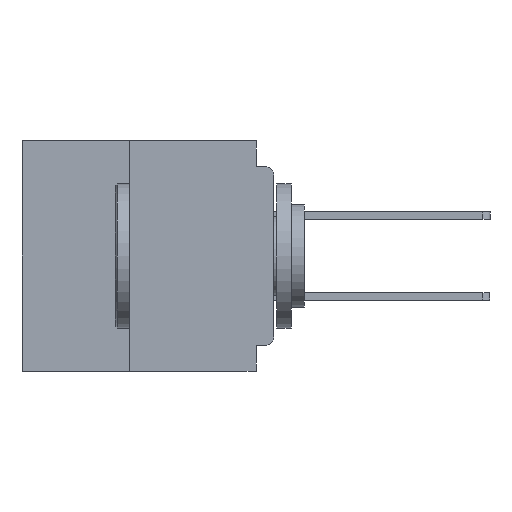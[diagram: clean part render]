
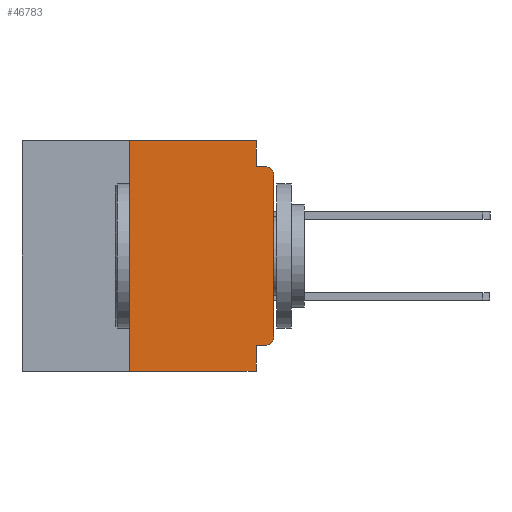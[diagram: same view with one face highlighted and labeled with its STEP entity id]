
A CAD part, left-side view. The second image highlights one B-rep face of the part: STEP entity #46783.
In plain terms, the highlighted planar face has unit normal (-1, 0, 0).
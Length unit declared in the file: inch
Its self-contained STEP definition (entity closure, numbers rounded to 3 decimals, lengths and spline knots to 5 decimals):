
#150 = VERTEX_POINT ( 'NONE', #36035 ) ;
#261 = ORIENTED_EDGE ( 'NONE', *, *, #5067, .T. ) ;
#636 = LINE ( 'NONE', #28807, #11610 ) ;
#663 = CARTESIAN_POINT ( 'NONE',  ( 0., 0.015, -0.355 ) ) ;
#1056 = CIRCLE ( 'NONE', #18691, 0.015 ) ;
#1163 = CIRCLE ( 'NONE', #52156, 0.015 ) ;
#1721 = ORIENTED_EDGE ( 'NONE', *, *, #18820, .F. ) ;
#1840 = LINE ( 'NONE', #54053, #12807 ) ;
#2618 = DIRECTION ( 'NONE',  ( 0., -1., 0. ) ) ;
#2851 = VERTEX_POINT ( 'NONE', #39978 ) ;
#3169 = DIRECTION ( 'NONE',  ( 0., 0., -1. ) ) ;
#3221 = VERTEX_POINT ( 'NONE', #18459 ) ;
#5067 = EDGE_CURVE ( 'NONE', #38964, #11904, #1056, .T. ) ;
#7493 = VECTOR ( 'NONE', #14672, 39.37008 ) ;
#8083 = LINE ( 'NONE', #48654, #31154 ) ;
#8415 = DIRECTION ( 'NONE',  ( 0., 0., -1. ) ) ;
#9556 = VERTEX_POINT ( 'NONE', #18477 ) ;
#10349 = EDGE_LOOP ( 'NONE', ( #28028, #261, #1721, #19710, #19076, #18080, #38736, #49837, #51034, #35666 ) ) ;
#10850 = EDGE_CURVE ( 'NONE', #9556, #2851, #44043, .T. ) ;
#11000 = VECTOR ( 'NONE', #44544, 39.37008 ) ;
#11610 = VECTOR ( 'NONE', #37905, 39.37008 ) ;
#11904 = VERTEX_POINT ( 'NONE', #25648 ) ;
#11950 = EDGE_CURVE ( 'NONE', #24018, #38964, #8083, .T. ) ;
#12476 = LINE ( 'NONE', #21723, #11000 ) ;
#12807 = VECTOR ( 'NONE', #8415, 39.37008 ) ;
#13900 = CARTESIAN_POINT ( 'NONE',  ( 0., 0.437, 0. ) ) ;
#14672 = DIRECTION ( 'NONE',  ( 0., 0., -1. ) ) ;
#15070 = VECTOR ( 'NONE', #2618, 39.37008 ) ;
#16464 = PLANE ( 'NONE',  #28823 ) ;
#16754 = VECTOR ( 'NONE', #18567, 39.37008 ) ;
#16931 = VERTEX_POINT ( 'NONE', #33832 ) ;
#18080 = ORIENTED_EDGE ( 'NONE', *, *, #25712, .F. ) ;
#18108 = DIRECTION ( 'NONE',  ( 0., 0., -1. ) ) ;
#18177 = DIRECTION ( 'NONE',  ( -1., 0., 0. ) ) ;
#18235 = CARTESIAN_POINT ( 'NONE',  ( 0., 0.015, -0.06 ) ) ;
#18459 = CARTESIAN_POINT ( 'NONE',  ( 0., 0.25, 0. ) ) ;
#18477 = CARTESIAN_POINT ( 'NONE',  ( 0., 0.031, 0. ) ) ;
#18567 = DIRECTION ( 'NONE',  ( 0., -1., 0. ) ) ;
#18691 = AXIS2_PLACEMENT_3D ( 'NONE', #18235, #18177, #18108 ) ;
#18820 = EDGE_CURVE ( 'NONE', #2851, #11904, #12476, .T. ) ;
#19076 = ORIENTED_EDGE ( 'NONE', *, *, #43792, .F. ) ;
#19710 = ORIENTED_EDGE ( 'NONE', *, *, #10850, .F. ) ;
#21723 = CARTESIAN_POINT ( 'NONE',  ( 0., 0., -0.045 ) ) ;
#21734 = CARTESIAN_POINT ( 'NONE',  ( 0., 0.031, -0.355 ) ) ;
#22183 = CARTESIAN_POINT ( 'NONE',  ( 0., 0., -0.06 ) ) ;
#24018 = VERTEX_POINT ( 'NONE', #51856 ) ;
#24829 = VERTEX_POINT ( 'NONE', #21734 ) ;
#25648 = CARTESIAN_POINT ( 'NONE',  ( 0., 0.015, -0.045 ) ) ;
#25712 = EDGE_CURVE ( 'NONE', #16931, #3221, #636, .T. ) ;
#26240 = DIRECTION ( 'NONE',  ( 0., 0., 1. ) ) ;
#26514 = DIRECTION ( 'NONE',  ( 0., 0., -1. ) ) ;
#27223 = EDGE_CURVE ( 'NONE', #24829, #150, #1840, .T. ) ;
#28028 = ORIENTED_EDGE ( 'NONE', *, *, #11950, .T. ) ;
#28807 = CARTESIAN_POINT ( 'NONE',  ( 0., 0.25, -0.4 ) ) ;
#28823 = AXIS2_PLACEMENT_3D ( 'NONE', #49145, #53748, #26514 ) ;
#30850 = DIRECTION ( 'NONE',  ( -1., 0., 0. ) ) ;
#31154 = VECTOR ( 'NONE', #26240, 39.37008 ) ;
#33461 = FACE_OUTER_BOUND ( 'NONE', #10349, .T. ) ;
#33832 = CARTESIAN_POINT ( 'NONE',  ( 0., 0.25, -0.4 ) ) ;
#35666 = ORIENTED_EDGE ( 'NONE', *, *, #51586, .T. ) ;
#36035 = CARTESIAN_POINT ( 'NONE',  ( 0., 0.031, -0.4 ) ) ;
#36520 = LINE ( 'NONE', #57551, #15070 ) ;
#37442 = CARTESIAN_POINT ( 'NONE',  ( 0., 0.031, 0. ) ) ;
#37905 = DIRECTION ( 'NONE',  ( 0., 0., 1. ) ) ;
#38736 = ORIENTED_EDGE ( 'NONE', *, *, #52542, .T. ) ;
#38964 = VERTEX_POINT ( 'NONE', #22183 ) ;
#39978 = CARTESIAN_POINT ( 'NONE',  ( 0., 0.031, -0.045 ) ) ;
#41183 = EDGE_CURVE ( 'NONE', #50142, #24829, #52018, .T. ) ;
#43792 = EDGE_CURVE ( 'NONE', #3221, #9556, #53115, .T. ) ;
#44043 = LINE ( 'NONE', #37442, #7493 ) ;
#44544 = DIRECTION ( 'NONE',  ( 0., -1., 0. ) ) ;
#46783 = ADVANCED_FACE ( 'NONE', ( #33461 ), #16464, .F. ) ;
#48124 = CARTESIAN_POINT ( 'NONE',  ( 0., 0., -0.355 ) ) ;
#48654 = CARTESIAN_POINT ( 'NONE',  ( 0., 0., 0. ) ) ;
#49145 = CARTESIAN_POINT ( 'NONE',  ( 0., 0.437, 0. ) ) ;
#49837 = ORIENTED_EDGE ( 'NONE', *, *, #27223, .F. ) ;
#50142 = VERTEX_POINT ( 'NONE', #663 ) ;
#50592 = VECTOR ( 'NONE', #52753, 39.37008 ) ;
#51034 = ORIENTED_EDGE ( 'NONE', *, *, #41183, .F. ) ;
#51586 = EDGE_CURVE ( 'NONE', #50142, #24018, #1163, .T. ) ;
#51856 = CARTESIAN_POINT ( 'NONE',  ( 0., 0., -0.34 ) ) ;
#52018 = LINE ( 'NONE', #48124, #50592 ) ;
#52156 = AXIS2_PLACEMENT_3D ( 'NONE', #58102, #30850, #3169 ) ;
#52542 = EDGE_CURVE ( 'NONE', #16931, #150, #36520, .T. ) ;
#52753 = DIRECTION ( 'NONE',  ( 0., 1., 0. ) ) ;
#53115 = LINE ( 'NONE', #13900, #16754 ) ;
#53748 = DIRECTION ( 'NONE',  ( 1., 0., 0. ) ) ;
#54053 = CARTESIAN_POINT ( 'NONE',  ( 0., 0.031, -0.4 ) ) ;
#57551 = CARTESIAN_POINT ( 'NONE',  ( 0., 0.437, -0.4 ) ) ;
#58102 = CARTESIAN_POINT ( 'NONE',  ( 0., 0.015, -0.34 ) ) ;
